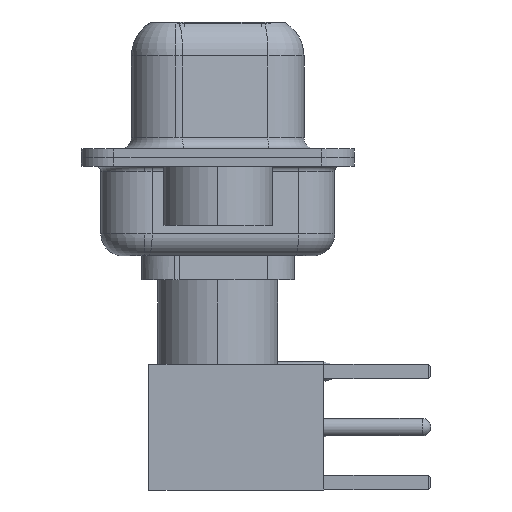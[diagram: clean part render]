
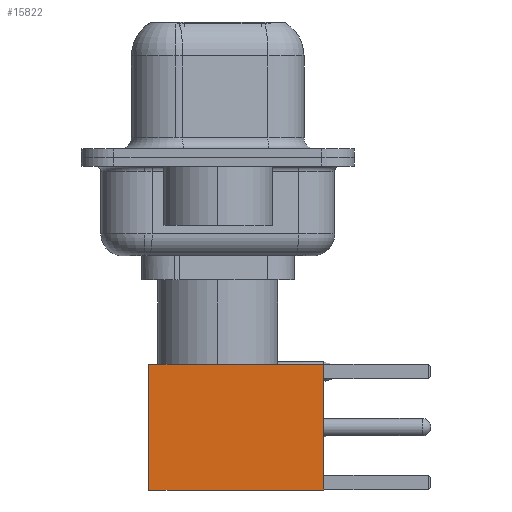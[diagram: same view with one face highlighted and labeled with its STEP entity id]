
A CAD part, left-side view. The second image highlights one B-rep face of the part: STEP entity #15822.
In plain terms, the highlighted face is planar.
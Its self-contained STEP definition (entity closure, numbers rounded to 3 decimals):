
#146 = EDGE_CURVE ( 'NONE', #6155, #8036, #5068, .T. ) ;
#1120 = LINE ( 'NONE', #20495, #12919 ) ;
#1677 = VECTOR ( 'NONE', #2799, 1000. ) ;
#2265 = VERTEX_POINT ( 'NONE', #15401 ) ;
#2420 = DIRECTION ( 'NONE',  ( 0., 0., -1. ) ) ;
#2799 = DIRECTION ( 'NONE',  ( -1., 0., 0. ) ) ;
#4695 = DIRECTION ( 'NONE',  ( 0., 0., 1. ) ) ;
#5068 = LINE ( 'NONE', #7105, #11486 ) ;
#6155 = VERTEX_POINT ( 'NONE', #19084 ) ;
#6304 = PLANE ( 'NONE',  #19976 ) ;
#7105 = CARTESIAN_POINT ( 'NONE',  ( 0., 2.875, 0. ) ) ;
#7759 = ORIENTED_EDGE ( 'NONE', *, *, #8762, .T. ) ;
#8036 = VERTEX_POINT ( 'NONE', #19093 ) ;
#8559 = EDGE_CURVE ( 'NONE', #18522, #8036, #1120, .T. ) ;
#8762 = EDGE_CURVE ( 'NONE', #2265, #6155, #9734, .T. ) ;
#9035 = ORIENTED_EDGE ( 'NONE', *, *, #8559, .F. ) ;
#9734 = LINE ( 'NONE', #13268, #20153 ) ;
#11486 = VECTOR ( 'NONE', #20026, 1000. ) ;
#12859 = EDGE_CURVE ( 'NONE', #2265, #18522, #15374, .T. ) ;
#12919 = VECTOR ( 'NONE', #2420, 1000. ) ;
#13268 = CARTESIAN_POINT ( 'NONE',  ( 2.875, 2.875, 0. ) ) ;
#14287 = CARTESIAN_POINT ( 'NONE',  ( -2.875, 2.875, 8. ) ) ;
#14467 = FACE_OUTER_BOUND ( 'NONE', #15167, .T. ) ;
#15167 = EDGE_LOOP ( 'NONE', ( #7759, #18947, #9035, #19131 ) ) ;
#15374 = LINE ( 'NONE', #15474, #1677 ) ;
#15401 = CARTESIAN_POINT ( 'NONE',  ( 2.875, 2.875, 8. ) ) ;
#15474 = CARTESIAN_POINT ( 'NONE',  ( 0., 2.875, 8. ) ) ;
#15822 = ADVANCED_FACE ( 'NONE', ( #14467 ), #6304, .T. ) ;
#16079 = CARTESIAN_POINT ( 'NONE',  ( 2.875, 2.875, 0. ) ) ;
#17803 = DIRECTION ( 'NONE',  ( 0., 0., -1. ) ) ;
#18522 = VERTEX_POINT ( 'NONE', #14287 ) ;
#18947 = ORIENTED_EDGE ( 'NONE', *, *, #146, .T. ) ;
#19084 = CARTESIAN_POINT ( 'NONE',  ( 2.875, 2.875, 0. ) ) ;
#19093 = CARTESIAN_POINT ( 'NONE',  ( -2.875, 2.875, 0. ) ) ;
#19131 = ORIENTED_EDGE ( 'NONE', *, *, #12859, .F. ) ;
#19976 = AXIS2_PLACEMENT_3D ( 'NONE', #16079, #20861, #4695 ) ;
#20026 = DIRECTION ( 'NONE',  ( -1., 0., 0. ) ) ;
#20153 = VECTOR ( 'NONE', #17803, 1000. ) ;
#20495 = CARTESIAN_POINT ( 'NONE',  ( -2.875, 2.875, 0. ) ) ;
#20861 = DIRECTION ( 'NONE',  ( 0., 1., 0. ) ) ;
